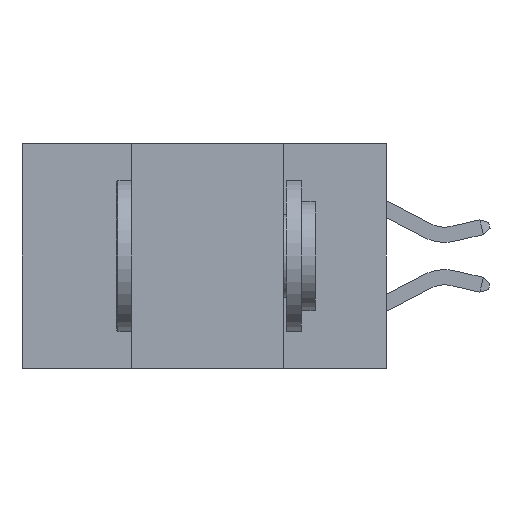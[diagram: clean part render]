
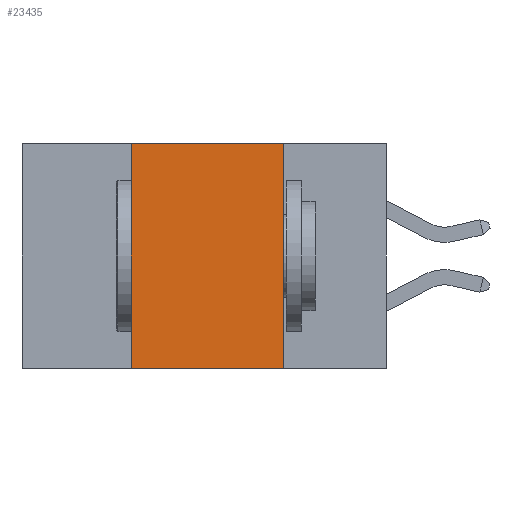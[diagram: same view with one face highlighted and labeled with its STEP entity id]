
A CAD part, left-side view. The second image highlights one B-rep face of the part: STEP entity #23435.
In plain terms, the highlighted planar face has unit normal (-1, 0, 0).
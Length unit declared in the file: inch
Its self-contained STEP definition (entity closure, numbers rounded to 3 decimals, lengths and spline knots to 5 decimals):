
#169 = PLANE ( 'NONE',  #3709 ) ;
#1537 = ORIENTED_EDGE ( 'NONE', *, *, #24407, .T. ) ;
#1725 = VERTEX_POINT ( 'NONE', #27890 ) ;
#2317 = CARTESIAN_POINT ( 'NONE',  ( 0., 0.6, 0. ) ) ;
#2409 = DIRECTION ( 'NONE',  ( 0., 0., -1. ) ) ;
#2414 = DIRECTION ( 'NONE',  ( 1., 0., 0. ) ) ;
#3247 = CARTESIAN_POINT ( 'NONE',  ( 0., 0.6, -0.37 ) ) ;
#3454 = LINE ( 'NONE', #3247, #19480 ) ;
#3709 = AXIS2_PLACEMENT_3D ( 'NONE', #2317, #2414, #17712 ) ;
#5221 = CARTESIAN_POINT ( 'NONE',  ( 0., 0.42, -0.37 ) ) ;
#8046 = ORIENTED_EDGE ( 'NONE', *, *, #8425, .F. ) ;
#8425 = EDGE_CURVE ( 'NONE', #16104, #1725, #27422, .T. ) ;
#8947 = VERTEX_POINT ( 'NONE', #20086 ) ;
#9141 = CARTESIAN_POINT ( 'NONE',  ( 0., 0.17, 0. ) ) ;
#9685 = VECTOR ( 'NONE', #18747, 39.37008 ) ;
#10356 = FACE_OUTER_BOUND ( 'NONE', #14436, .T. ) ;
#10678 = VERTEX_POINT ( 'NONE', #9141 ) ;
#12021 = CARTESIAN_POINT ( 'NONE',  ( 0., 0.42, -0.37 ) ) ;
#13351 = EDGE_CURVE ( 'NONE', #10678, #8947, #14765, .T. ) ;
#13392 = VECTOR ( 'NONE', #2409, 39.37008 ) ;
#13406 = CARTESIAN_POINT ( 'NONE',  ( 0., 0.17, -0.37 ) ) ;
#14314 = DIRECTION ( 'NONE',  ( 0., 0., 1. ) ) ;
#14436 = EDGE_LOOP ( 'NONE', ( #20354, #25329, #8046, #1537 ) ) ;
#14765 = LINE ( 'NONE', #13406, #13392 ) ;
#15517 = LINE ( 'NONE', #22994, #9685 ) ;
#16104 = VERTEX_POINT ( 'NONE', #5221 ) ;
#17712 = DIRECTION ( 'NONE',  ( 0., 0., -1. ) ) ;
#18747 = DIRECTION ( 'NONE',  ( 0., -1., 0. ) ) ;
#19480 = VECTOR ( 'NONE', #27059, 39.37008 ) ;
#20086 = CARTESIAN_POINT ( 'NONE',  ( 0., 0.17, -0.37 ) ) ;
#20354 = ORIENTED_EDGE ( 'NONE', *, *, #13351, .F. ) ;
#21149 = VECTOR ( 'NONE', #14314, 39.37008 ) ;
#22982 = EDGE_CURVE ( 'NONE', #1725, #10678, #15517, .T. ) ;
#22994 = CARTESIAN_POINT ( 'NONE',  ( 0., 0.6, 0. ) ) ;
#23435 = ADVANCED_FACE ( 'NONE', ( #10356 ), #169, .F. ) ;
#24407 = EDGE_CURVE ( 'NONE', #16104, #8947, #3454, .T. ) ;
#25329 = ORIENTED_EDGE ( 'NONE', *, *, #22982, .F. ) ;
#27059 = DIRECTION ( 'NONE',  ( 0., -1., 0. ) ) ;
#27422 = LINE ( 'NONE', #12021, #21149 ) ;
#27890 = CARTESIAN_POINT ( 'NONE',  ( 0., 0.42, 0. ) ) ;
